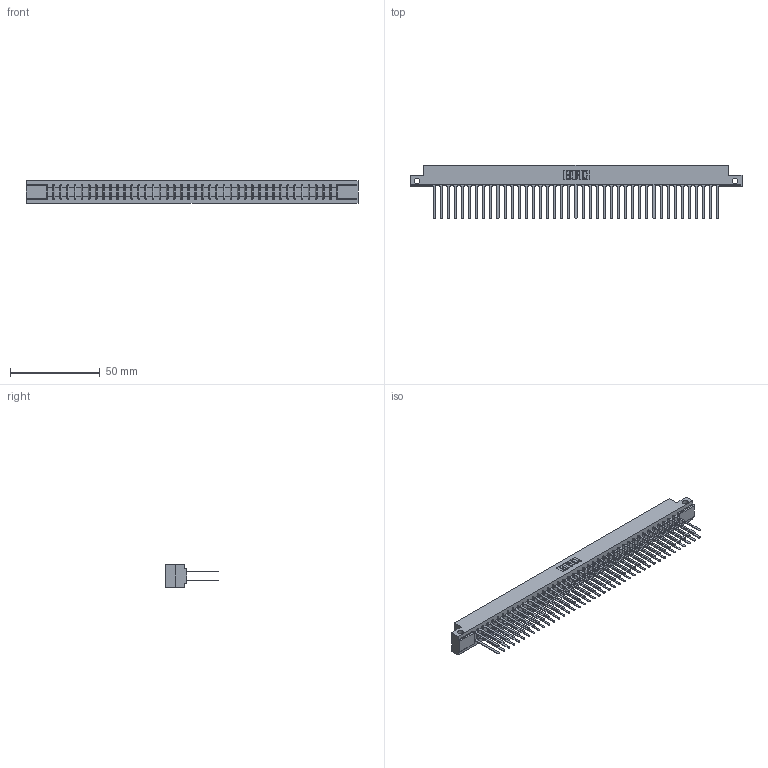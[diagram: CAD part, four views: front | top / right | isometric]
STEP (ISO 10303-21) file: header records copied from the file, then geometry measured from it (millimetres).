
FILE_DESCRIPTION (( 'STEP AP203' ), '1' );
FILE_NAME ('357-082-440-212.STEP', '2020-10-04T09:57:26', ( '' ), ( '' ), 'SwSTEP 2.0', 'SolidWorks 2020', '' );
FILE_SCHEMA (( 'CONFIG_CONTROL_DESIGN' ));
Length unit declared in the file: inch
Products named in the file (3): 307-290-001_540; 307 Part_.128 Dia Side Mounting Holes; 357-082-440-212
Assembly tree (83 placements, depth 2):
  357-082-440-212
    307 Part_.128 Dia Side Mounting Holes
    307-290-001_540  x82
Bounding box: 185.47 x 30 x 12.7 mm (x, y, z)
Volume: 20031.3 mm3; surface area: 27209.9 mm2
Topology: 83 solids, 83 shells, 3932 faces, 10983 edges, 7098 vertices
Faces by surface type: plane 2612, cylinder 1236, sphere 84
Entity records: 36554 total; most frequent: CARTESIAN_POINT 5977, ORIENTED_EDGE 5922, DIRECTION 5855, EDGE_CURVE 2961, VECTOR 2271, LINE 2271, VERTEX_POINT 1914, AXIS2_PLACEMENT_3D 1792
